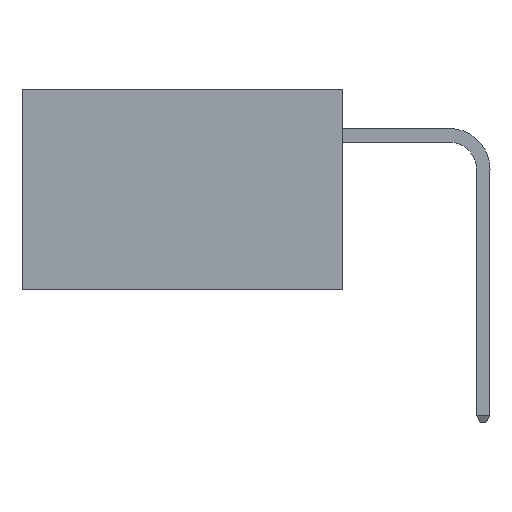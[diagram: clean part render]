
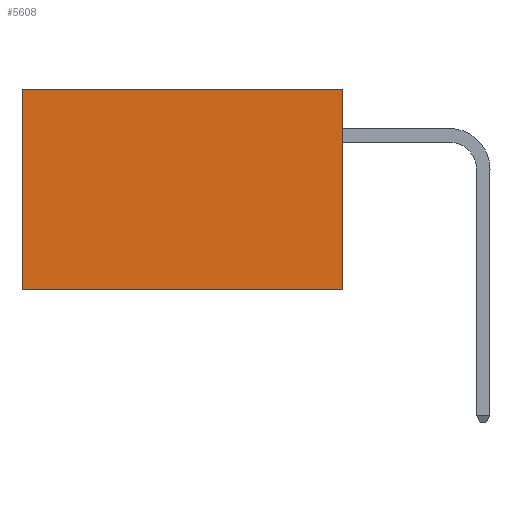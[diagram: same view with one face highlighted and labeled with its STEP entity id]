
A CAD part, left-side view. The second image highlights one B-rep face of the part: STEP entity #5608.
In plain terms, the highlighted planar face has unit normal (-1, 0, 0).
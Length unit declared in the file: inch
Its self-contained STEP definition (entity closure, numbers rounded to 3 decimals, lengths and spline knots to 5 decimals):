
#97 = PLANE ( 'NONE',  #2338 ) ;
#425 = EDGE_CURVE ( 'NONE', #3635, #2004, #1862, .T. ) ;
#631 = DIRECTION ( 'NONE',  ( 0., 1., 0. ) ) ;
#900 = CARTESIAN_POINT ( 'NONE',  ( 0.277, 0., -0.37 ) ) ;
#1780 = CARTESIAN_POINT ( 'NONE',  ( 0.277, 0., -0.37 ) ) ;
#1862 = LINE ( 'NONE', #1780, #9704 ) ;
#2004 = VERTEX_POINT ( 'NONE', #6219 ) ;
#2338 = AXIS2_PLACEMENT_3D ( 'NONE', #900, #9937, #9890 ) ;
#2756 = CARTESIAN_POINT ( 'NONE',  ( 0.277, 0.59, 0. ) ) ;
#3325 = VERTEX_POINT ( 'NONE', #9508 ) ;
#3433 = DIRECTION ( 'NONE',  ( 0., 0., -1. ) ) ;
#3635 = VERTEX_POINT ( 'NONE', #8428 ) ;
#4007 = EDGE_CURVE ( 'NONE', #2004, #3325, #9615, .T. ) ;
#4108 = LINE ( 'NONE', #9814, #5795 ) ;
#4175 = EDGE_CURVE ( 'NONE', #9160, #3325, #4108, .T. ) ;
#4850 = DIRECTION ( 'NONE',  ( 0., 1., 0. ) ) ;
#5202 = DIRECTION ( 'NONE',  ( 0., 0., -1. ) ) ;
#5378 = VECTOR ( 'NONE', #631, 39.37008 ) ;
#5608 = ADVANCED_FACE ( 'NONE', ( #7907 ), #97, .F. ) ;
#5649 = LINE ( 'NONE', #9788, #5378 ) ;
#5795 = VECTOR ( 'NONE', #3433, 39.37008 ) ;
#6219 = CARTESIAN_POINT ( 'NONE',  ( 0.277, 0., -0.37 ) ) ;
#7112 = ORIENTED_EDGE ( 'NONE', *, *, #7576, .T. ) ;
#7186 = ORIENTED_EDGE ( 'NONE', *, *, #425, .F. ) ;
#7247 = ORIENTED_EDGE ( 'NONE', *, *, #4007, .F. ) ;
#7277 = ORIENTED_EDGE ( 'NONE', *, *, #4175, .T. ) ;
#7576 = EDGE_CURVE ( 'NONE', #3635, #9160, #5649, .T. ) ;
#7907 = FACE_OUTER_BOUND ( 'NONE', #9772, .T. ) ;
#7956 = VECTOR ( 'NONE', #4850, 39.37008 ) ;
#8428 = CARTESIAN_POINT ( 'NONE',  ( 0.277, 0., 0. ) ) ;
#9160 = VERTEX_POINT ( 'NONE', #2756 ) ;
#9508 = CARTESIAN_POINT ( 'NONE',  ( 0.277, 0.59, -0.37 ) ) ;
#9615 = LINE ( 'NONE', #9825, #7956 ) ;
#9704 = VECTOR ( 'NONE', #5202, 39.37008 ) ;
#9772 = EDGE_LOOP ( 'NONE', ( #7277, #7247, #7186, #7112 ) ) ;
#9788 = CARTESIAN_POINT ( 'NONE',  ( 0.277, 0., 0. ) ) ;
#9814 = CARTESIAN_POINT ( 'NONE',  ( 0.277, 0.59, -0.37 ) ) ;
#9825 = CARTESIAN_POINT ( 'NONE',  ( 0.277, 0., -0.37 ) ) ;
#9890 = DIRECTION ( 'NONE',  ( 0., 0., -1. ) ) ;
#9937 = DIRECTION ( 'NONE',  ( 1., 0., 0. ) ) ;
